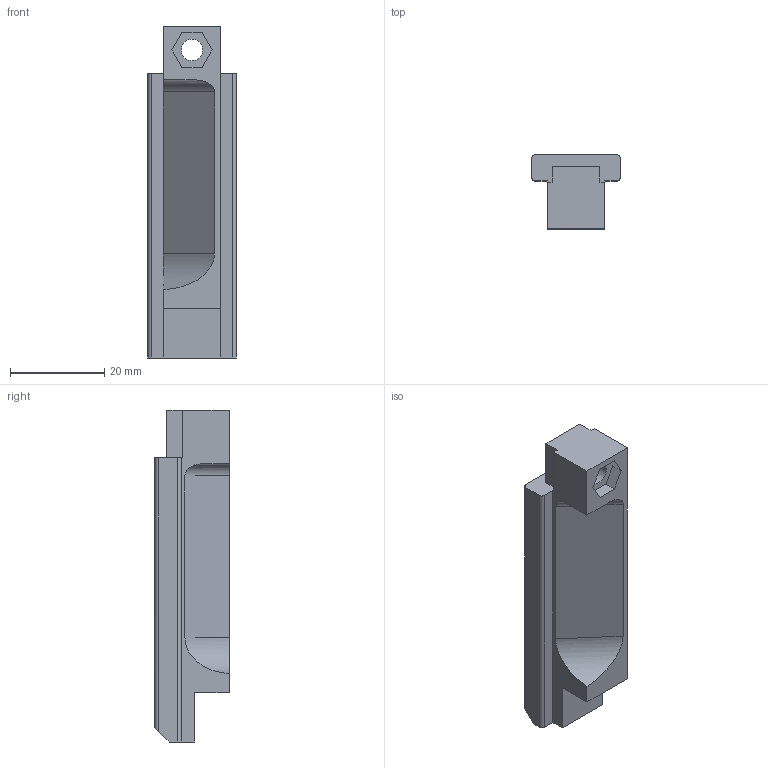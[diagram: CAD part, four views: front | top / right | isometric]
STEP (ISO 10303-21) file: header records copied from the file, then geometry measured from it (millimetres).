
FILE_DESCRIPTION (( 'STEP AP214' ), '1' );
FILE_NAME ('Charging Handle Body.STEP', '2022-03-05T02:06:58', ( '' ), ( '' ), 'SwSTEP 2.0', 'SolidWorks 2020', '' );
FILE_SCHEMA (( 'AUTOMOTIVE_DESIGN' ));
Length unit declared in the file: inch
Products named in the file (1): Charging Handle Body
Bounding box: 18.69 x 15.8 x 70.36 mm (x, y, z)
Volume: 11823.1 mm3; surface area: 4859 mm2
Topology: 1 solids, 1 shells, 65 faces, 177 edges, 118 vertices
Faces by surface type: plane 41, bspline 16, cylinder 8
Entity records: 2449 total; most frequent: CARTESIAN_POINT 875, ORIENTED_EDGE 354, DIRECTION 249, EDGE_CURVE 177, VECTOR 129, LINE 129, VERTEX_POINT 118, EDGE_LOOP 71
